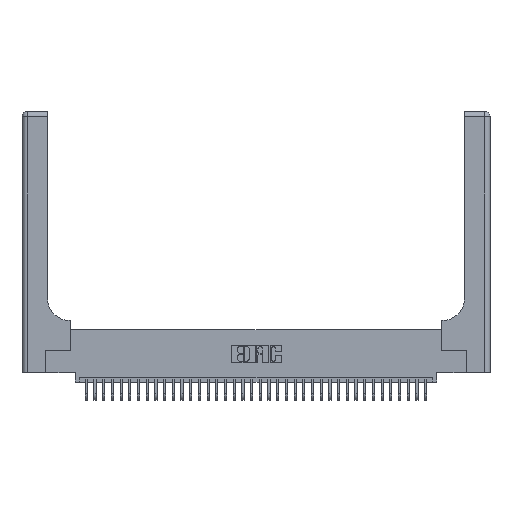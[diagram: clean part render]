
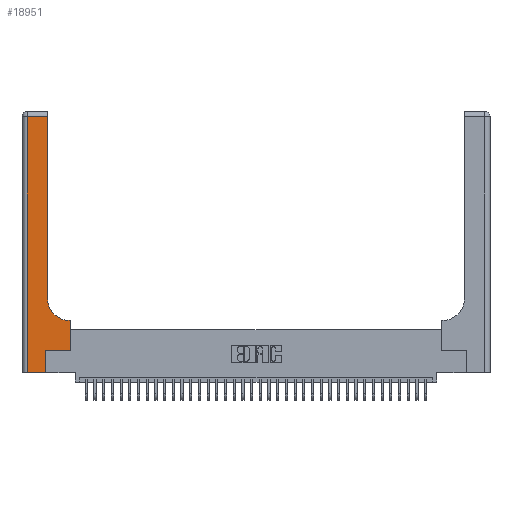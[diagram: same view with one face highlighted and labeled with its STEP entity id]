
A CAD part, top view. The second image highlights one B-rep face of the part: STEP entity #18951.
In plain terms, the highlighted planar face has unit normal (0, 0, 1).
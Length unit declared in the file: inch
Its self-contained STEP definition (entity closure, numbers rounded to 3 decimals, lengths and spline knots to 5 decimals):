
#157 = VERTEX_POINT ( 'NONE', #22869 ) ;
#446 = EDGE_CURVE ( 'NONE', #16227, #32302, #31878, .T. ) ;
#475 = FACE_OUTER_BOUND ( 'NONE', #22085, .T. ) ;
#489 = ORIENTED_EDGE ( 'NONE', *, *, #32244, .T. ) ;
#739 = ORIENTED_EDGE ( 'NONE', *, *, #12800, .T. ) ;
#956 = CARTESIAN_POINT ( 'NONE',  ( 0., 0., 0.37 ) ) ;
#2272 = ORIENTED_EDGE ( 'NONE', *, *, #2614, .T. ) ;
#2418 = CARTESIAN_POINT ( 'NONE',  ( 0.269, 0., 0.37 ) ) ;
#2614 = EDGE_CURVE ( 'NONE', #20739, #16227, #13431, .T. ) ;
#2626 = CARTESIAN_POINT ( 'NONE',  ( 0.269, 0.25, 0.37 ) ) ;
#2909 = CARTESIAN_POINT ( 'NONE',  ( 0.06, 3., 0.37 ) ) ;
#5079 = VECTOR ( 'NONE', #27705, 39.37008 ) ;
#5234 = DIRECTION ( 'NONE',  ( 0., 0., -1. ) ) ;
#5371 = DIRECTION ( 'NONE',  ( 0., 1., 0. ) ) ;
#5747 = AXIS2_PLACEMENT_3D ( 'NONE', #17440, #32219, #17319 ) ;
#6523 = EDGE_CURVE ( 'NONE', #34943, #12169, #22559, .T. ) ;
#9391 = DIRECTION ( 'NONE',  ( 0., -1., 0. ) ) ;
#10281 = VECTOR ( 'NONE', #11369, 39.37008 ) ;
#10407 = ORIENTED_EDGE ( 'NONE', *, *, #15795, .T. ) ;
#10541 = CARTESIAN_POINT ( 'NONE',  ( 0.2915, 3., 0.37 ) ) ;
#10701 = DIRECTION ( 'NONE',  ( -1., 0., 0. ) ) ;
#10765 = EDGE_CURVE ( 'NONE', #12169, #20739, #12901, .T. ) ;
#11151 = CARTESIAN_POINT ( 'NONE',  ( 0.06, 2.94, 0.37 ) ) ;
#11197 = VECTOR ( 'NONE', #5371, 39.37008 ) ;
#11264 = CARTESIAN_POINT ( 'NONE',  ( 0.269, 0., 0.37 ) ) ;
#11369 = DIRECTION ( 'NONE',  ( 1., 0., 0. ) ) ;
#11463 = ORIENTED_EDGE ( 'NONE', *, *, #35413, .T. ) ;
#12169 = VERTEX_POINT ( 'NONE', #28604 ) ;
#12800 = EDGE_CURVE ( 'NONE', #16255, #30726, #13603, .T. ) ;
#12901 = CIRCLE ( 'NONE', #27258, 0.25 ) ;
#13431 = LINE ( 'NONE', #10541, #25133 ) ;
#13603 = LINE ( 'NONE', #2626, #10281 ) ;
#13815 = VECTOR ( 'NONE', #21389, 39.37008 ) ;
#14867 = CARTESIAN_POINT ( 'NONE',  ( 0.269, 0.25, 0.37 ) ) ;
#15795 = EDGE_CURVE ( 'NONE', #30726, #34943, #33427, .T. ) ;
#16227 = VERTEX_POINT ( 'NONE', #23600 ) ;
#16255 = VERTEX_POINT ( 'NONE', #14867 ) ;
#16809 = LINE ( 'NONE', #956, #5079 ) ;
#17319 = DIRECTION ( 'NONE',  ( -1., 0., 0. ) ) ;
#17359 = VECTOR ( 'NONE', #10701, 39.37008 ) ;
#17440 = CARTESIAN_POINT ( 'NONE',  ( 0., 3., 0.37 ) ) ;
#17970 = CARTESIAN_POINT ( 'NONE',  ( 0.5585, 0.25, 0.37 ) ) ;
#18839 = CARTESIAN_POINT ( 'NONE',  ( 0.2915, 0.85, 0.37 ) ) ;
#18951 = ADVANCED_FACE ( 'NONE', ( #475 ), #26606, .F. ) ;
#19336 = DIRECTION ( 'NONE',  ( 0., 1., 0. ) ) ;
#19396 = DIRECTION ( 'NONE',  ( -1., 0., 0. ) ) ;
#20028 = ORIENTED_EDGE ( 'NONE', *, *, #23690, .T. ) ;
#20739 = VERTEX_POINT ( 'NONE', #18839 ) ;
#21389 = DIRECTION ( 'NONE',  ( 0., 1., 0. ) ) ;
#22085 = EDGE_LOOP ( 'NONE', ( #2272, #29070, #11463, #20028, #489, #739, #10407, #36308, #38353 ) ) ;
#22559 = LINE ( 'NONE', #37293, #27664 ) ;
#22822 = LINE ( 'NONE', #2909, #23763 ) ;
#22856 = CARTESIAN_POINT ( 'NONE',  ( 0., 2.94, 0.37 ) ) ;
#22869 = CARTESIAN_POINT ( 'NONE',  ( 0.06, 0., 0.37 ) ) ;
#23272 = CARTESIAN_POINT ( 'NONE',  ( 0.5415, 0.85, 0.37 ) ) ;
#23600 = CARTESIAN_POINT ( 'NONE',  ( 0.2915, 2.94, 0.37 ) ) ;
#23690 = EDGE_CURVE ( 'NONE', #157, #30024, #16809, .T. ) ;
#23763 = VECTOR ( 'NONE', #9391, 39.37008 ) ;
#24279 = CARTESIAN_POINT ( 'NONE',  ( 0.5585, 0.25, 0.37 ) ) ;
#25133 = VECTOR ( 'NONE', #19336, 39.37008 ) ;
#26305 = DIRECTION ( 'NONE',  ( 1., 0., 0. ) ) ;
#26606 = PLANE ( 'NONE',  #5747 ) ;
#27258 = AXIS2_PLACEMENT_3D ( 'NONE', #23272, #5234, #26305 ) ;
#27546 = CARTESIAN_POINT ( 'NONE',  ( 0.5585, 0.6, 0.37 ) ) ;
#27664 = VECTOR ( 'NONE', #19396, 39.37008 ) ;
#27705 = DIRECTION ( 'NONE',  ( 1., 0., 0. ) ) ;
#28604 = CARTESIAN_POINT ( 'NONE',  ( 0.5415, 0.6, 0.37 ) ) ;
#29070 = ORIENTED_EDGE ( 'NONE', *, *, #446, .T. ) ;
#29420 = LINE ( 'NONE', #2418, #11197 ) ;
#30024 = VERTEX_POINT ( 'NONE', #11264 ) ;
#30726 = VERTEX_POINT ( 'NONE', #17970 ) ;
#31878 = LINE ( 'NONE', #22856, #17359 ) ;
#32219 = DIRECTION ( 'NONE',  ( 0., 0., -1. ) ) ;
#32244 = EDGE_CURVE ( 'NONE', #30024, #16255, #29420, .T. ) ;
#32302 = VERTEX_POINT ( 'NONE', #11151 ) ;
#33427 = LINE ( 'NONE', #24279, #13815 ) ;
#34943 = VERTEX_POINT ( 'NONE', #27546 ) ;
#35413 = EDGE_CURVE ( 'NONE', #32302, #157, #22822, .T. ) ;
#36308 = ORIENTED_EDGE ( 'NONE', *, *, #6523, .T. ) ;
#37293 = CARTESIAN_POINT ( 'NONE',  ( 0.2915, 0.6, 0.37 ) ) ;
#38353 = ORIENTED_EDGE ( 'NONE', *, *, #10765, .T. ) ;
